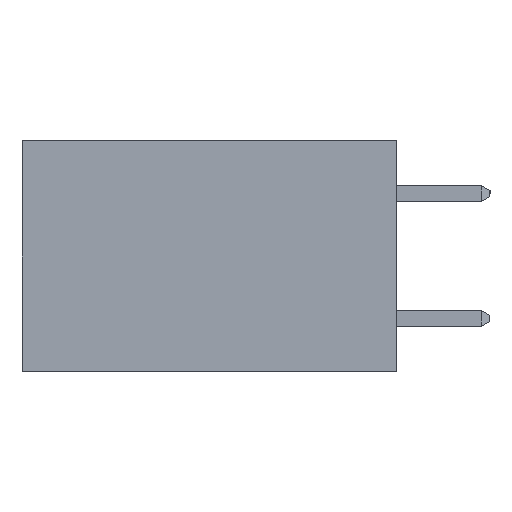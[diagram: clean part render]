
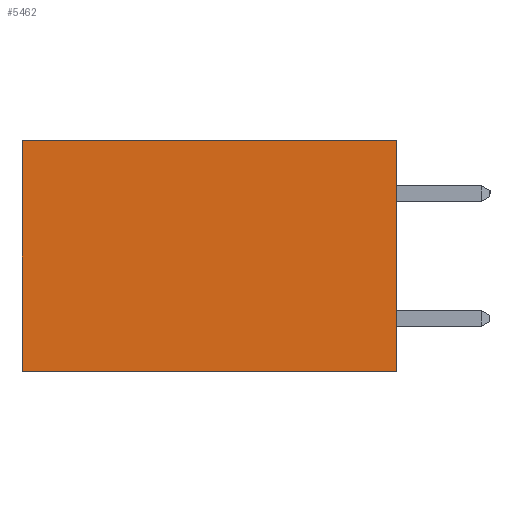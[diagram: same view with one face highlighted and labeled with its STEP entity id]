
A CAD part, left-side view. The second image highlights one B-rep face of the part: STEP entity #5462.
In plain terms, the highlighted planar face has unit normal (-1, 0, 0).
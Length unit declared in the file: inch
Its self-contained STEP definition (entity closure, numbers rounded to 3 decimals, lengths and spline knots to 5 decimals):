
#125 = CARTESIAN_POINT ( 'NONE',  ( 0.2615, 0., -0.37 ) ) ;
#1082 = ORIENTED_EDGE ( 'NONE', *, *, #18808, .F. ) ;
#1308 = LINE ( 'NONE', #12473, #23049 ) ;
#1700 = ORIENTED_EDGE ( 'NONE', *, *, #20434, .T. ) ;
#2004 = DIRECTION ( 'NONE',  ( 0., 1., 0. ) ) ;
#3044 = EDGE_CURVE ( 'NONE', #5060, #17438, #12428, .T. ) ;
#3366 = DIRECTION ( 'NONE',  ( 1., 0., 0. ) ) ;
#4653 = ORIENTED_EDGE ( 'NONE', *, *, #3044, .F. ) ;
#5060 = VERTEX_POINT ( 'NONE', #7450 ) ;
#5328 = VECTOR ( 'NONE', #18175, 39.37008 ) ;
#5462 = ADVANCED_FACE ( 'NONE', ( #21972 ), #21745, .F. ) ;
#7187 = DIRECTION ( 'NONE',  ( 0., 0., -1. ) ) ;
#7450 = CARTESIAN_POINT ( 'NONE',  ( 0.2615, 0., -0.37 ) ) ;
#8981 = EDGE_LOOP ( 'NONE', ( #1700, #4653, #1082, #11011 ) ) ;
#9656 = AXIS2_PLACEMENT_3D ( 'NONE', #125, #3366, #7187 ) ;
#9677 = CARTESIAN_POINT ( 'NONE',  ( 0.2615, 0., 0. ) ) ;
#10731 = LINE ( 'NONE', #13008, #5328 ) ;
#11011 = ORIENTED_EDGE ( 'NONE', *, *, #13503, .T. ) ;
#12065 = DIRECTION ( 'NONE',  ( 0., 1., 0. ) ) ;
#12428 = LINE ( 'NONE', #14340, #22996 ) ;
#12473 = CARTESIAN_POINT ( 'NONE',  ( 0.2615, 0.6, -0.37 ) ) ;
#12588 = DIRECTION ( 'NONE',  ( 0., 0., -1. ) ) ;
#12890 = CARTESIAN_POINT ( 'NONE',  ( 0.2615, 0.6, -0.37 ) ) ;
#13008 = CARTESIAN_POINT ( 'NONE',  ( 0.2615, 0., -0.37 ) ) ;
#13503 = EDGE_CURVE ( 'NONE', #23575, #19295, #15204, .T. ) ;
#14340 = CARTESIAN_POINT ( 'NONE',  ( 0.2615, 0., -0.37 ) ) ;
#15204 = LINE ( 'NONE', #9677, #19034 ) ;
#15940 = CARTESIAN_POINT ( 'NONE',  ( 0.2615, 0., 0. ) ) ;
#16709 = CARTESIAN_POINT ( 'NONE',  ( 0.2615, 0.6, 0. ) ) ;
#17438 = VERTEX_POINT ( 'NONE', #12890 ) ;
#18175 = DIRECTION ( 'NONE',  ( 0., 0., -1. ) ) ;
#18808 = EDGE_CURVE ( 'NONE', #23575, #5060, #10731, .T. ) ;
#19034 = VECTOR ( 'NONE', #2004, 39.37008 ) ;
#19295 = VERTEX_POINT ( 'NONE', #16709 ) ;
#20434 = EDGE_CURVE ( 'NONE', #19295, #17438, #1308, .T. ) ;
#21745 = PLANE ( 'NONE',  #9656 ) ;
#21972 = FACE_OUTER_BOUND ( 'NONE', #8981, .T. ) ;
#22996 = VECTOR ( 'NONE', #12065, 39.37008 ) ;
#23049 = VECTOR ( 'NONE', #12588, 39.37008 ) ;
#23575 = VERTEX_POINT ( 'NONE', #15940 ) ;
